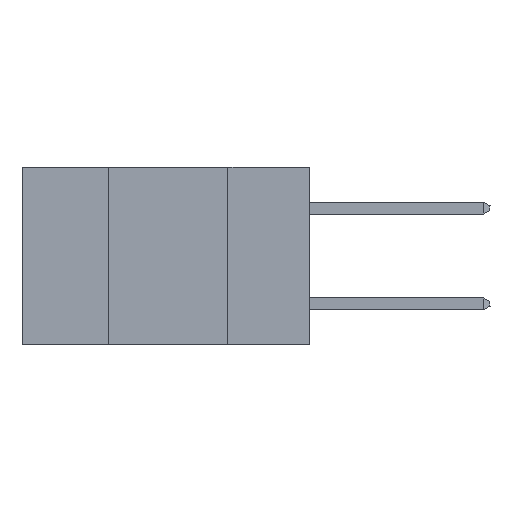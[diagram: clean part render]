
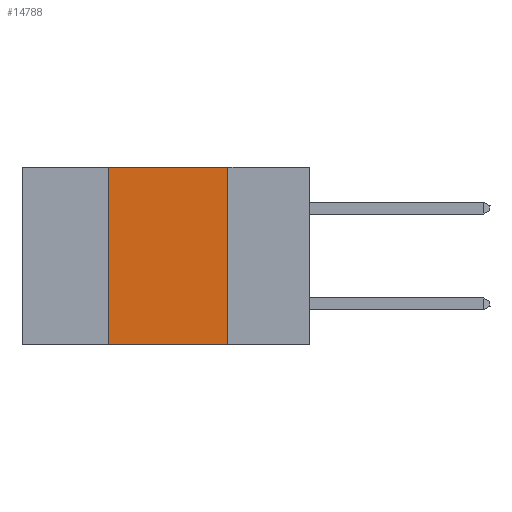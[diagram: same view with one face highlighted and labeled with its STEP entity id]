
A CAD part, left-side view. The second image highlights one B-rep face of the part: STEP entity #14788.
In plain terms, the highlighted planar face has unit normal (-1, 0, 0).
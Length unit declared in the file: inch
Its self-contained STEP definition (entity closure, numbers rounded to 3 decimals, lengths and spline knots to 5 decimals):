
#125 = EDGE_CURVE ( 'NONE', #27657, #1895, #8687, .T. ) ;
#1895 = VERTEX_POINT ( 'NONE', #2533 ) ;
#2143 = CARTESIAN_POINT ( 'NONE',  ( 0., 0.42, 0. ) ) ;
#2533 = CARTESIAN_POINT ( 'NONE',  ( 0., 0.17, 0. ) ) ;
#3304 = VECTOR ( 'NONE', #32498, 39.37008 ) ;
#3361 = LINE ( 'NONE', #2143, #3753 ) ;
#3370 = DIRECTION ( 'NONE',  ( 0., -1., 0. ) ) ;
#3753 = VECTOR ( 'NONE', #15479, 39.37008 ) ;
#4331 = VERTEX_POINT ( 'NONE', #15357 ) ;
#6883 = LINE ( 'NONE', #26100, #7325 ) ;
#7325 = VECTOR ( 'NONE', #33880, 39.37008 ) ;
#8687 = LINE ( 'NONE', #16262, #3304 ) ;
#10345 = CARTESIAN_POINT ( 'NONE',  ( 0., 0.42, 0. ) ) ;
#14135 = EDGE_LOOP ( 'NONE', ( #23122, #17952, #18410, #33231 ) ) ;
#14196 = VERTEX_POINT ( 'NONE', #17242 ) ;
#14788 = ADVANCED_FACE ( 'NONE', ( #27210 ), #22499, .F. ) ;
#15357 = CARTESIAN_POINT ( 'NONE',  ( 0., 0.17, -0.37 ) ) ;
#15479 = DIRECTION ( 'NONE',  ( 0., 0., 1. ) ) ;
#16262 = CARTESIAN_POINT ( 'NONE',  ( 0., 0.6, 0. ) ) ;
#17242 = CARTESIAN_POINT ( 'NONE',  ( 0., 0.42, -0.37 ) ) ;
#17952 = ORIENTED_EDGE ( 'NONE', *, *, #125, .F. ) ;
#18410 = ORIENTED_EDGE ( 'NONE', *, *, #22949, .F. ) ;
#18801 = EDGE_CURVE ( 'NONE', #1895, #4331, #6883, .T. ) ;
#21776 = DIRECTION ( 'NONE',  ( 1., 0., 0. ) ) ;
#21891 = DIRECTION ( 'NONE',  ( 0., 0., -1. ) ) ;
#22499 = PLANE ( 'NONE',  #30790 ) ;
#22949 = EDGE_CURVE ( 'NONE', #14196, #27657, #3361, .T. ) ;
#23122 = ORIENTED_EDGE ( 'NONE', *, *, #18801, .F. ) ;
#26100 = CARTESIAN_POINT ( 'NONE',  ( 0., 0.17, 0. ) ) ;
#26554 = LINE ( 'NONE', #32850, #31950 ) ;
#27210 = FACE_OUTER_BOUND ( 'NONE', #14135, .T. ) ;
#27657 = VERTEX_POINT ( 'NONE', #10345 ) ;
#28559 = CARTESIAN_POINT ( 'NONE',  ( 0., 0.6, 0. ) ) ;
#29998 = EDGE_CURVE ( 'NONE', #14196, #4331, #26554, .T. ) ;
#30790 = AXIS2_PLACEMENT_3D ( 'NONE', #28559, #21776, #21891 ) ;
#31950 = VECTOR ( 'NONE', #3370, 39.37008 ) ;
#32498 = DIRECTION ( 'NONE',  ( 0., -1., 0. ) ) ;
#32850 = CARTESIAN_POINT ( 'NONE',  ( 0., 0.6, -0.37 ) ) ;
#33231 = ORIENTED_EDGE ( 'NONE', *, *, #29998, .T. ) ;
#33880 = DIRECTION ( 'NONE',  ( 0., 0., -1. ) ) ;
